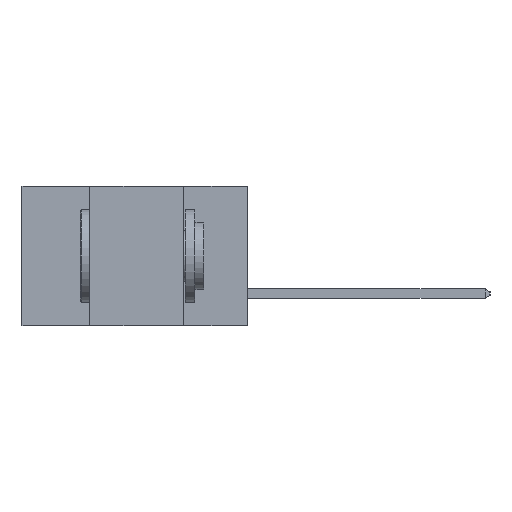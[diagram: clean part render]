
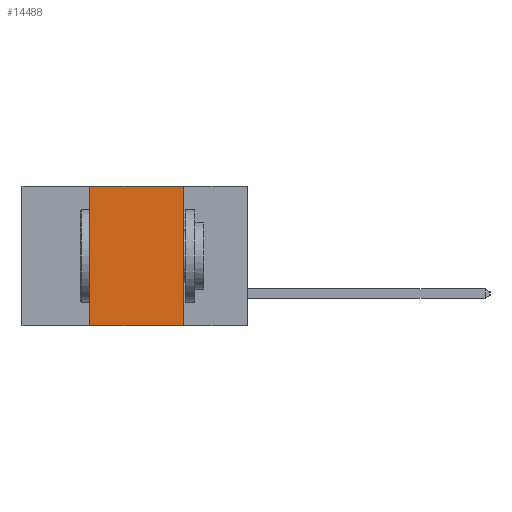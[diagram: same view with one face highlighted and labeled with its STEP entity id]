
A CAD part, left-side view. The second image highlights one B-rep face of the part: STEP entity #14488.
In plain terms, the highlighted planar face has unit normal (-1, 0, 0).
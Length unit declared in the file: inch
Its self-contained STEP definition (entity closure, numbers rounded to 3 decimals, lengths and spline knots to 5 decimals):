
#479 = DIRECTION ( 'NONE',  ( 0., -1., 0. ) ) ;
#632 = CARTESIAN_POINT ( 'NONE',  ( 0., 0.17, -0.37 ) ) ;
#764 = ORIENTED_EDGE ( 'NONE', *, *, #1760, .F. ) ;
#1226 = VERTEX_POINT ( 'NONE', #4528 ) ;
#1522 = CARTESIAN_POINT ( 'NONE',  ( 0., 0.42, 0. ) ) ;
#1760 = EDGE_CURVE ( 'NONE', #1226, #8523, #12094, .T. ) ;
#2500 = FACE_OUTER_BOUND ( 'NONE', #6725, .T. ) ;
#4157 = AXIS2_PLACEMENT_3D ( 'NONE', #11946, #4229, #13276 ) ;
#4229 = DIRECTION ( 'NONE',  ( 1., 0., 0. ) ) ;
#4498 = ORIENTED_EDGE ( 'NONE', *, *, #13400, .T. ) ;
#4528 = CARTESIAN_POINT ( 'NONE',  ( 0., 0.17, 0. ) ) ;
#4689 = ORIENTED_EDGE ( 'NONE', *, *, #11641, .F. ) ;
#6725 = EDGE_LOOP ( 'NONE', ( #764, #4689, #9937, #4498 ) ) ;
#6955 = VERTEX_POINT ( 'NONE', #8456 ) ;
#6972 = CARTESIAN_POINT ( 'NONE',  ( 0., 0.42, -0.37 ) ) ;
#8294 = DIRECTION ( 'NONE',  ( 0., 0., 1. ) ) ;
#8456 = CARTESIAN_POINT ( 'NONE',  ( 0., 0.42, -0.37 ) ) ;
#8523 = VERTEX_POINT ( 'NONE', #632 ) ;
#8791 = DIRECTION ( 'NONE',  ( 0., -1., 0. ) ) ;
#8859 = VECTOR ( 'NONE', #479, 39.37008 ) ;
#9252 = VECTOR ( 'NONE', #8294, 39.37008 ) ;
#9387 = PLANE ( 'NONE',  #4157 ) ;
#9882 = VECTOR ( 'NONE', #8791, 39.37008 ) ;
#9937 = ORIENTED_EDGE ( 'NONE', *, *, #13377, .F. ) ;
#10107 = CARTESIAN_POINT ( 'NONE',  ( 0., 0.17, -0.37 ) ) ;
#10164 = DIRECTION ( 'NONE',  ( 0., 0., -1. ) ) ;
#11641 = EDGE_CURVE ( 'NONE', #11903, #1226, #14119, .T. ) ;
#11903 = VERTEX_POINT ( 'NONE', #1522 ) ;
#11946 = CARTESIAN_POINT ( 'NONE',  ( 0., 0.6, 0. ) ) ;
#12094 = LINE ( 'NONE', #10107, #15532 ) ;
#12249 = LINE ( 'NONE', #14738, #8859 ) ;
#12654 = LINE ( 'NONE', #6972, #9252 ) ;
#13276 = DIRECTION ( 'NONE',  ( 0., 0., -1. ) ) ;
#13377 = EDGE_CURVE ( 'NONE', #6955, #11903, #12654, .T. ) ;
#13400 = EDGE_CURVE ( 'NONE', #6955, #8523, #12249, .T. ) ;
#14119 = LINE ( 'NONE', #15186, #9882 ) ;
#14488 = ADVANCED_FACE ( 'NONE', ( #2500 ), #9387, .F. ) ;
#14738 = CARTESIAN_POINT ( 'NONE',  ( 0., 0.6, -0.37 ) ) ;
#15186 = CARTESIAN_POINT ( 'NONE',  ( 0., 0.6, 0. ) ) ;
#15532 = VECTOR ( 'NONE', #10164, 39.37008 ) ;
